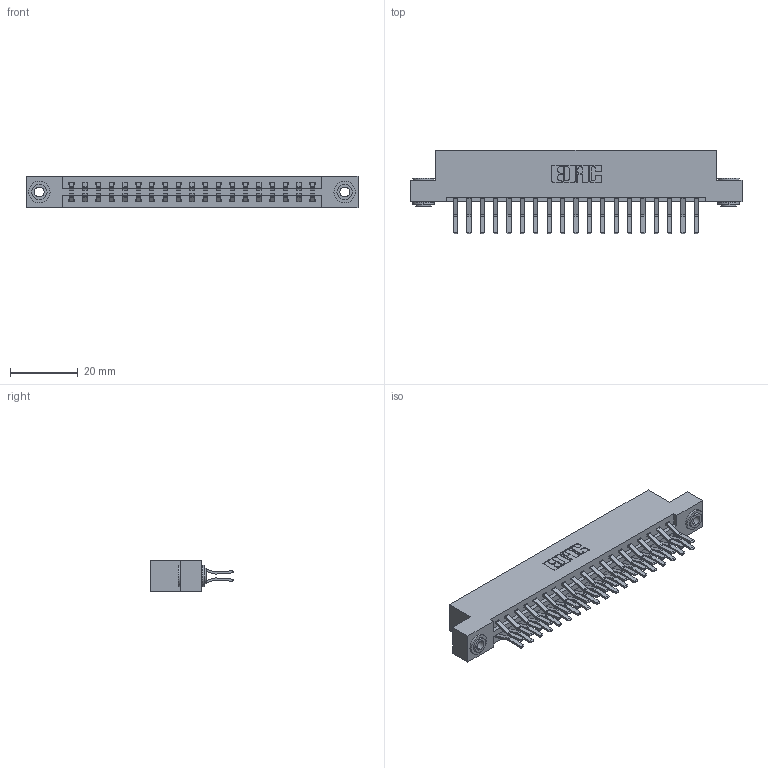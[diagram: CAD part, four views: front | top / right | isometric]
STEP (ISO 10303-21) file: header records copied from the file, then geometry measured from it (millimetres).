
FILE_DESCRIPTION (( 'STEP AP203' ), '1' );
FILE_NAME ('337-038-560-203.STEP', '2018-08-08T06:17:46', ( '' ), ( '' ), 'SwSTEP 2.0', 'SolidWorks 2016', '' );
FILE_SCHEMA (( 'CONFIG_CONTROL_DESIGN' ));
Length unit declared in the file: inch
Products named in the file (4): 345-250-002_345-250-002-102; 337-038-560-203; 337 Part_Flush Mounting Lugs - 0.156 Dia-TH; 345-292-001_560 Tail
Assembly tree (41 placements, depth 2):
  337-038-560-203
    337 Part_Flush Mounting Lugs - 0.156 Dia-TH
    345-292-001_560 Tail  x38
    345-250-002_345-250-002-102  x2
Bounding box: 98.3 x 24.78 x 9.4 mm (x, y, z)
Volume: 10321.7 mm3; surface area: 12390.6 mm2
Topology: 41 solids, 41 shells, 2280 faces, 6733 edges, 4434 vertices
Faces by surface type: plane 1524, cylinder 748, cone 8
Entity records: 18444 total; most frequent: CARTESIAN_POINT 3101, ORIENTED_EDGE 3030, DIRECTION 2717, EDGE_CURVE 1515, LINE 1359, VECTOR 1359, VERTEX_POINT 1006, AXIS2_PLACEMENT_3D 679
